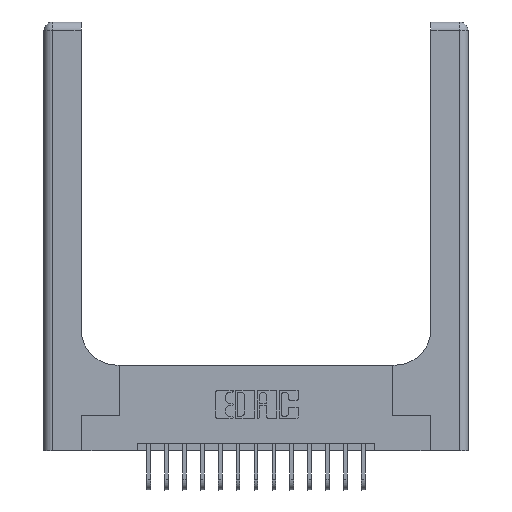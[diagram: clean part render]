
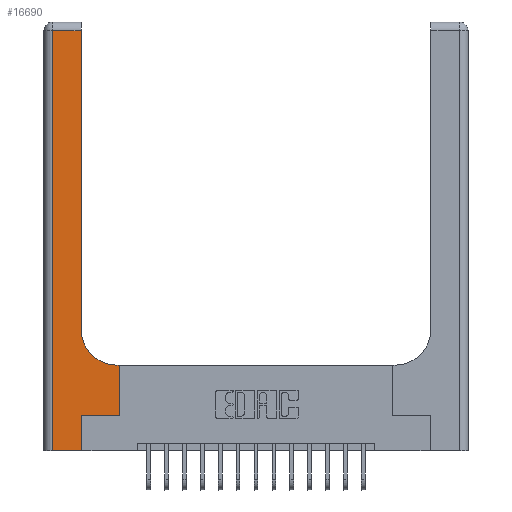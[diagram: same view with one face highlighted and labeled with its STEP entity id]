
A CAD part, top view. The second image highlights one B-rep face of the part: STEP entity #16690.
In plain terms, the highlighted planar face has unit normal (0, 0, 1).
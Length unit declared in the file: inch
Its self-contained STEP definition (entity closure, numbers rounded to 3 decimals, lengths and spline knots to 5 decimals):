
#359 = CARTESIAN_POINT ( 'NONE',  ( 0.06, 0., 0.37 ) ) ;
#470 = LINE ( 'NONE', #5741, #546 ) ;
#546 = VECTOR ( 'NONE', #13115, 39.37008 ) ;
#696 = CARTESIAN_POINT ( 'NONE',  ( 0.265, 0.25, 0.37 ) ) ;
#950 = DIRECTION ( 'NONE',  ( 0., 0., -1. ) ) ;
#1087 = VERTEX_POINT ( 'NONE', #359 ) ;
#1594 = LINE ( 'NONE', #1769, #2455 ) ;
#1769 = CARTESIAN_POINT ( 'NONE',  ( 0.26, 0.6, 0.37 ) ) ;
#1808 = EDGE_CURVE ( 'NONE', #2399, #8212, #470, .T. ) ;
#1857 = CARTESIAN_POINT ( 'NONE',  ( 0., 0., 0.37 ) ) ;
#2012 = AXIS2_PLACEMENT_3D ( 'NONE', #10541, #13163, #13522 ) ;
#2393 = DIRECTION ( 'NONE',  ( 1., 0., 0. ) ) ;
#2399 = VERTEX_POINT ( 'NONE', #15125 ) ;
#2455 = VECTOR ( 'NONE', #11009, 39.37008 ) ;
#2563 = CARTESIAN_POINT ( 'NONE',  ( 0.51, 0.85, 0.37 ) ) ;
#2846 = ORIENTED_EDGE ( 'NONE', *, *, #16076, .T. ) ;
#2998 = VERTEX_POINT ( 'NONE', #5595 ) ;
#3206 = VECTOR ( 'NONE', #5640, 39.37008 ) ;
#3639 = DIRECTION ( 'NONE',  ( 1., 0., 0. ) ) ;
#3752 = ORIENTED_EDGE ( 'NONE', *, *, #15341, .T. ) ;
#3794 = ORIENTED_EDGE ( 'NONE', *, *, #1808, .T. ) ;
#3927 = DIRECTION ( 'NONE',  ( 0., 1., 0. ) ) ;
#4208 = ORIENTED_EDGE ( 'NONE', *, *, #14520, .T. ) ;
#4723 = ORIENTED_EDGE ( 'NONE', *, *, #5299, .T. ) ;
#4775 = CARTESIAN_POINT ( 'NONE',  ( 0., 2.94, 0.37 ) ) ;
#4801 = LINE ( 'NONE', #1857, #11612 ) ;
#4945 = ORIENTED_EDGE ( 'NONE', *, *, #13089, .T. ) ;
#5101 = VERTEX_POINT ( 'NONE', #7129 ) ;
#5299 = EDGE_CURVE ( 'NONE', #11789, #9294, #6502, .T. ) ;
#5378 = AXIS2_PLACEMENT_3D ( 'NONE', #2563, #950, #3639 ) ;
#5421 = EDGE_CURVE ( 'NONE', #5101, #11789, #9562, .T. ) ;
#5503 = CARTESIAN_POINT ( 'NONE',  ( 0.528, 0.25, 0.37 ) ) ;
#5595 = CARTESIAN_POINT ( 'NONE',  ( 0.528, 0.6, 0.37 ) ) ;
#5640 = DIRECTION ( 'NONE',  ( 0., -1., 0. ) ) ;
#5741 = CARTESIAN_POINT ( 'NONE',  ( 0.26, 3., 0.37 ) ) ;
#6092 = CARTESIAN_POINT ( 'NONE',  ( 0.06, 2.94, 0.37 ) ) ;
#6502 = LINE ( 'NONE', #696, #16575 ) ;
#6696 = ORIENTED_EDGE ( 'NONE', *, *, #5421, .T. ) ;
#6699 = VERTEX_POINT ( 'NONE', #6092 ) ;
#6845 = CARTESIAN_POINT ( 'NONE',  ( 0.51, 0.6, 0.37 ) ) ;
#7129 = CARTESIAN_POINT ( 'NONE',  ( 0.265, 0., 0.37 ) ) ;
#8181 = CARTESIAN_POINT ( 'NONE',  ( 0.26, 2.94, 0.37 ) ) ;
#8212 = VERTEX_POINT ( 'NONE', #8181 ) ;
#8299 = VECTOR ( 'NONE', #16512, 39.37008 ) ;
#8450 = EDGE_CURVE ( 'NONE', #8212, #6699, #11765, .T. ) ;
#8979 = DIRECTION ( 'NONE',  ( -1., 0., 0. ) ) ;
#9294 = VERTEX_POINT ( 'NONE', #5503 ) ;
#9447 = VECTOR ( 'NONE', #3927, 39.37008 ) ;
#9562 = LINE ( 'NONE', #12189, #9447 ) ;
#10263 = DIRECTION ( 'NONE',  ( 1., 0., 0. ) ) ;
#10541 = CARTESIAN_POINT ( 'NONE',  ( 0., 3., 0.37 ) ) ;
#10890 = CARTESIAN_POINT ( 'NONE',  ( 0.265, 0.25, 0.37 ) ) ;
#11009 = DIRECTION ( 'NONE',  ( -1., 0., 0. ) ) ;
#11533 = ORIENTED_EDGE ( 'NONE', *, *, #8450, .T. ) ;
#11612 = VECTOR ( 'NONE', #10263, 39.37008 ) ;
#11765 = LINE ( 'NONE', #4775, #13844 ) ;
#11789 = VERTEX_POINT ( 'NONE', #10890 ) ;
#12189 = CARTESIAN_POINT ( 'NONE',  ( 0.265, 0., 0.37 ) ) ;
#12529 = LINE ( 'NONE', #16846, #8299 ) ;
#12558 = CIRCLE ( 'NONE', #5378, 0.25 ) ;
#12573 = LINE ( 'NONE', #12662, #3206 ) ;
#12662 = CARTESIAN_POINT ( 'NONE',  ( 0.06, 3., 0.37 ) ) ;
#12851 = ORIENTED_EDGE ( 'NONE', *, *, #13241, .T. ) ;
#13089 = EDGE_CURVE ( 'NONE', #2998, #15205, #1594, .T. ) ;
#13115 = DIRECTION ( 'NONE',  ( 0., 1., 0. ) ) ;
#13163 = DIRECTION ( 'NONE',  ( 0., 0., -1. ) ) ;
#13241 = EDGE_CURVE ( 'NONE', #1087, #5101, #4801, .T. ) ;
#13275 = EDGE_LOOP ( 'NONE', ( #3794, #11533, #2846, #12851, #6696, #4723, #3752, #4945, #4208 ) ) ;
#13341 = FACE_OUTER_BOUND ( 'NONE', #13275, .T. ) ;
#13522 = DIRECTION ( 'NONE',  ( -1., 0., 0. ) ) ;
#13844 = VECTOR ( 'NONE', #8979, 39.37008 ) ;
#14520 = EDGE_CURVE ( 'NONE', #15205, #2399, #12558, .T. ) ;
#15125 = CARTESIAN_POINT ( 'NONE',  ( 0.26, 0.85, 0.37 ) ) ;
#15205 = VERTEX_POINT ( 'NONE', #6845 ) ;
#15341 = EDGE_CURVE ( 'NONE', #9294, #2998, #12529, .T. ) ;
#15825 = PLANE ( 'NONE',  #2012 ) ;
#16076 = EDGE_CURVE ( 'NONE', #6699, #1087, #12573, .T. ) ;
#16512 = DIRECTION ( 'NONE',  ( 0., 1., 0. ) ) ;
#16575 = VECTOR ( 'NONE', #2393, 39.37008 ) ;
#16690 = ADVANCED_FACE ( 'NONE', ( #13341 ), #15825, .F. ) ;
#16846 = CARTESIAN_POINT ( 'NONE',  ( 0.528, 0.25, 0.37 ) ) ;
